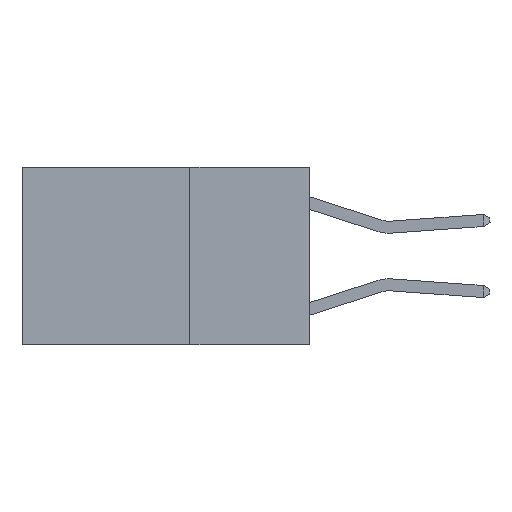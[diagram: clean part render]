
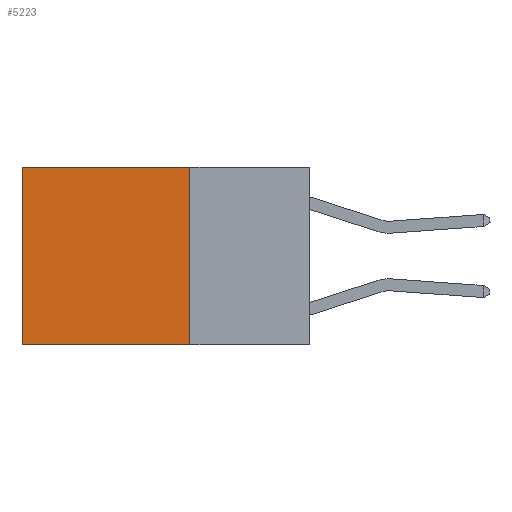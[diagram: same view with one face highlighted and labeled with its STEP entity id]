
A CAD part, left-side view. The second image highlights one B-rep face of the part: STEP entity #5223.
In plain terms, the highlighted planar face has unit normal (-1, 0, 0).
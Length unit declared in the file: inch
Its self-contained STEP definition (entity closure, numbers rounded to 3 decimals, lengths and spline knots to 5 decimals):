
#74 = CARTESIAN_POINT ( 'NONE',  ( 0.2625, 0.25, 0. ) ) ;
#142 = ORIENTED_EDGE ( 'NONE', *, *, #8295, .F. ) ;
#490 = FACE_OUTER_BOUND ( 'NONE', #1895, .T. ) ;
#491 = DIRECTION ( 'NONE',  ( 1., 0., 0. ) ) ;
#769 = CARTESIAN_POINT ( 'NONE',  ( 0.2625, 0.6, 0. ) ) ;
#1400 = LINE ( 'NONE', #74, #8603 ) ;
#1503 = DIRECTION ( 'NONE',  ( 0., 1., 0. ) ) ;
#1504 = VERTEX_POINT ( 'NONE', #2292 ) ;
#1895 = EDGE_LOOP ( 'NONE', ( #7212, #142, #8837, #7574 ) ) ;
#2292 = CARTESIAN_POINT ( 'NONE',  ( 0.2625, 0.25, 0. ) ) ;
#2468 = LINE ( 'NONE', #3931, #4102 ) ;
#2484 = DIRECTION ( 'NONE',  ( 0., 0., -1. ) ) ;
#2789 = VECTOR ( 'NONE', #2484, 39.37008 ) ;
#2809 = EDGE_CURVE ( 'NONE', #4792, #7329, #4628, .T. ) ;
#3673 = VERTEX_POINT ( 'NONE', #5555 ) ;
#3931 = CARTESIAN_POINT ( 'NONE',  ( 0.2625, 0.25, 0. ) ) ;
#4026 = PLANE ( 'NONE',  #6897 ) ;
#4102 = VECTOR ( 'NONE', #6782, 39.37008 ) ;
#4273 = CARTESIAN_POINT ( 'NONE',  ( 0.2625, 0.25, -0.37 ) ) ;
#4628 = LINE ( 'NONE', #6090, #2789 ) ;
#4733 = CARTESIAN_POINT ( 'NONE',  ( 0.2625, 0.25, 0. ) ) ;
#4763 = VECTOR ( 'NONE', #1503, 39.37008 ) ;
#4792 = VERTEX_POINT ( 'NONE', #769 ) ;
#5101 = DIRECTION ( 'NONE',  ( 0., 0., -1. ) ) ;
#5223 = ADVANCED_FACE ( 'NONE', ( #490 ), #4026, .F. ) ;
#5412 = CARTESIAN_POINT ( 'NONE',  ( 0.2625, 0.6, -0.37 ) ) ;
#5519 = DIRECTION ( 'NONE',  ( 0., 0., -1. ) ) ;
#5555 = CARTESIAN_POINT ( 'NONE',  ( 0.2625, 0.25, -0.37 ) ) ;
#5640 = EDGE_CURVE ( 'NONE', #1504, #3673, #1400, .T. ) ;
#6090 = CARTESIAN_POINT ( 'NONE',  ( 0.2625, 0.6, 0. ) ) ;
#6305 = EDGE_CURVE ( 'NONE', #1504, #4792, #2468, .T. ) ;
#6782 = DIRECTION ( 'NONE',  ( 0., 1., 0. ) ) ;
#6897 = AXIS2_PLACEMENT_3D ( 'NONE', #4733, #491, #5519 ) ;
#7212 = ORIENTED_EDGE ( 'NONE', *, *, #2809, .T. ) ;
#7329 = VERTEX_POINT ( 'NONE', #5412 ) ;
#7574 = ORIENTED_EDGE ( 'NONE', *, *, #6305, .T. ) ;
#8287 = LINE ( 'NONE', #4273, #4763 ) ;
#8295 = EDGE_CURVE ( 'NONE', #3673, #7329, #8287, .T. ) ;
#8603 = VECTOR ( 'NONE', #5101, 39.37008 ) ;
#8837 = ORIENTED_EDGE ( 'NONE', *, *, #5640, .F. ) ;
